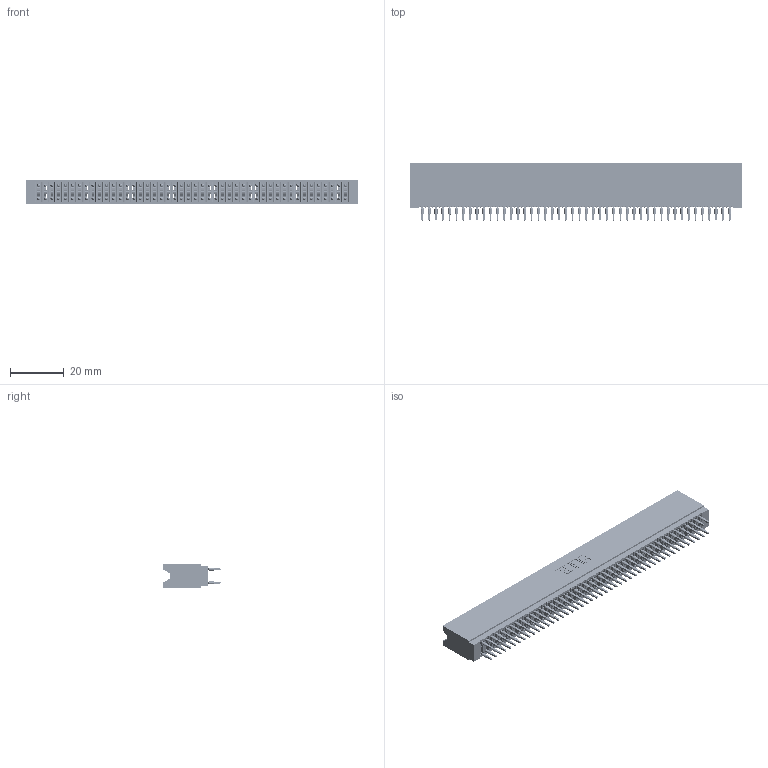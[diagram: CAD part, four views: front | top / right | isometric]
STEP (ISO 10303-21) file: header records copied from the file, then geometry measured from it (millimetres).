
FILE_DESCRIPTION (( 'STEP AP203' ), '1' );
FILE_NAME ('745-092-560-206.STEP', '2026-02-26T22:42:45', ( '' ), ( '' ), 'SwSTEP 2.0', 'SolidWorks 2023', '' );
FILE_SCHEMA (( 'CONFIG_CONTROL_DESIGN' ));
Length unit declared in the file: millimetre
Products named in the file (3): 745 Part_Insulator Option - 06; 745-292-001_560; 745-092-560-206
Assembly tree (93 placements, depth 2):
  745-092-560-206
    745 Part_Insulator Option - 06
    745-292-001_560  x92
Bounding box: 123.44 x 21.22 x 8.89 mm (x, y, z)
Volume: 11410.6 mm3; surface area: 24768 mm2
Topology: 93 solids, 93 shells, 9158 faces, 25054 edges, 15904 vertices
Faces by surface type: plane 4748, cylinder 2018, bspline 1840, torus 552
Entity records: 77239 total; most frequent: CARTESIAN_POINT 13900, ORIENTED_EDGE 13344, DIRECTION 11658, EDGE_CURVE 6672, LINE 6206, VECTOR 6206, VERTEX_POINT 4256, AXIS2_PLACEMENT_3D 2726
